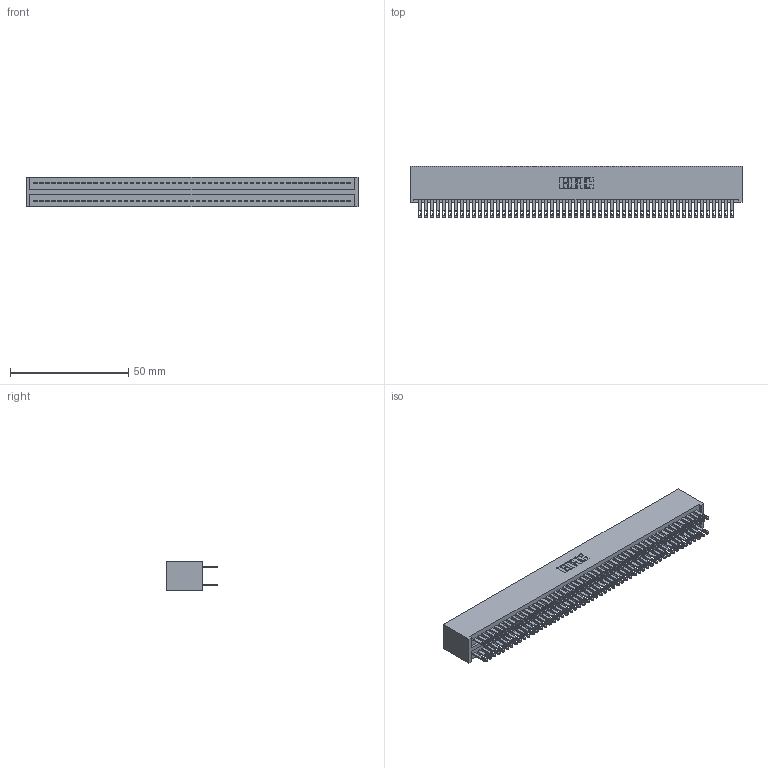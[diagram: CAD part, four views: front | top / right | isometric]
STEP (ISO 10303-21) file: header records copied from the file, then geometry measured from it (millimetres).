
FILE_DESCRIPTION (( 'STEP AP203' ), '1' );
FILE_NAME ('325-106-500-201.STEP', '2020-02-25T07:09:15', ( '' ), ( '' ), 'SwSTEP 2.0', 'SolidWorks 2016', '' );
FILE_SCHEMA (( 'CONFIG_CONTROL_DESIGN' ));
Length unit declared in the file: inch
Products named in the file (3): 325-292-001_325-293-100; 325 Part_Lugless; 325-106-500-201
Assembly tree (107 placements, depth 2):
  325-106-500-201
    325 Part_Lugless
    325-292-001_325-293-100  x106
Bounding box: 140.26 x 21.84 x 12.45 mm (x, y, z)
Volume: 19135.6 mm3; surface area: 25191.3 mm2
Topology: 107 solids, 107 shells, 5194 faces, 15869 edges, 10578 vertices
Faces by surface type: plane 3246, cylinder 1948
Entity records: 32327 total; most frequent: CARTESIAN_POINT 5342, ORIENTED_EDGE 5278, DIRECTION 4539, EDGE_CURVE 2639, LINE 2515, VECTOR 2515, VERTEX_POINT 1758, AXIS2_PLACEMENT_3D 1012
